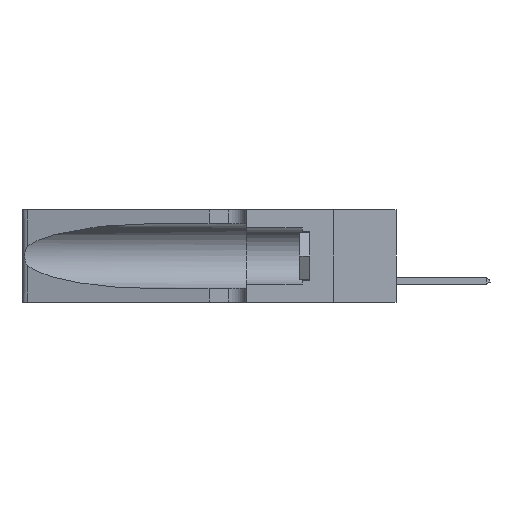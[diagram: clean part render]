
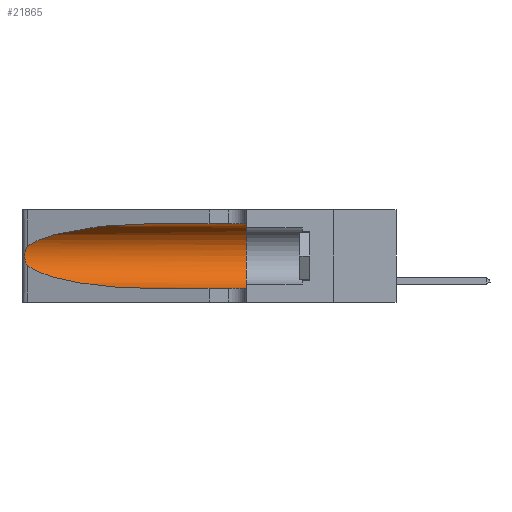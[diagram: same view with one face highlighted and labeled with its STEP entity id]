
A CAD part, left-side view. The second image highlights one B-rep face of the part: STEP entity #21865.
In plain terms, the highlighted cylindrical face has radius 3.308 mm (diameter 6.617 mm), a partial arc.
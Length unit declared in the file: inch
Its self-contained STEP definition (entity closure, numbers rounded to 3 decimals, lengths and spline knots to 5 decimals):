
#190 = AXIS2_PLACEMENT_3D ( 'NONE', #4617, #20242, #4769 ) ;
#362 = CARTESIAN_POINT ( 'NONE',  ( 0.1305, 0.72297, 0.31525 ) ) ;
#919 = CARTESIAN_POINT ( 'NONE',  ( 0.1305, 0.72297, 0.31525 ) ) ;
#1406 = CARTESIAN_POINT ( 'NONE',  ( 0.25487, 1.22718, 0.14631 ) ) ;
#1492 = CARTESIAN_POINT ( 'NONE',  ( 0.26017, 1.23833, 0.17102 ) ) ;
#1553 = CARTESIAN_POINT ( 'NONE',  ( 0.25639, 1.23186, 0.15144 ) ) ;
#1636 = FACE_OUTER_BOUND ( 'NONE', #13879, .T. ) ;
#1815 =( BOUNDED_CURVE ( )  B_SPLINE_CURVE ( 3, ( #362, #12248, #20667, #10382 ),
 .UNSPECIFIED., .F., .T. ) 
 B_SPLINE_CURVE_WITH_KNOTS ( ( 4, 4 ),
 ( 1.5708, 2.84003 ),
 .UNSPECIFIED. ) 
 CURVE ( )  GEOMETRIC_REPRESENTATION_ITEM ( )  RATIONAL_B_SPLINE_CURVE ( ( 1., 0.87, 0.87, 1. ) ) 
 REPRESENTATION_ITEM ( '' )  );
#1851 = VERTEX_POINT ( 'NONE', #919 ) ;
#1918 = ORIENTED_EDGE ( 'NONE', *, *, #15136, .T. ) ;
#2074 = CARTESIAN_POINT ( 'NONE',  ( 0.1305, 1.61858, 0.05475 ) ) ;
#2279 = ORIENTED_EDGE ( 'NONE', *, *, #8762, .F. ) ;
#3175 = B_SPLINE_CURVE_WITH_KNOTS ( 'NONE', 3,
 ( #19698, #7088, #13924, #10709, #17206, #14140, #3721, #17667, #1492, #15080, #20320, #1553, #10096, #13503 ),
 .UNSPECIFIED., .F., .F.,
 ( 4, 2, 2, 2, 2, 2, 4 ),
 ( 0., 0.00027, 0.00053, 0.00107, 0.0016, 0.00187, 0.00214 ),
 .UNSPECIFIED. ) ;
#3478 = VERTEX_POINT ( 'NONE', #22032 ) ;
#3645 = LINE ( 'NONE', #2074, #8427 ) ;
#3721 = CARTESIAN_POINT ( 'NONE',  ( 0.26075, 1.23896, 0.19203 ) ) ;
#4617 = CARTESIAN_POINT ( 'NONE',  ( 0.1305, 0.35, 0.185 ) ) ;
#4769 = DIRECTION ( 'NONE',  ( 0., 0., 1. ) ) ;
#4831 = ORIENTED_EDGE ( 'NONE', *, *, #8500, .T. ) ;
#4931 = DIRECTION ( 'NONE',  ( 0., -1., 0. ) ) ;
#5470 = ORIENTED_EDGE ( 'NONE', *, *, #7664, .T. ) ;
#5628 = CYLINDRICAL_SURFACE ( 'NONE', #19272, 0.13025 ) ;
#5633 = CARTESIAN_POINT ( 'NONE',  ( 0.1305, 1.61858, 0.31525 ) ) ;
#6149 = VERTEX_POINT ( 'NONE', #20934 ) ;
#7088 = CARTESIAN_POINT ( 'NONE',  ( 0.25555, 1.22994, 0.2215 ) ) ;
#7664 = EDGE_CURVE ( 'NONE', #10566, #19313, #8110, .T. ) ;
#7800 = CARTESIAN_POINT ( 'NONE',  ( 0.1305, 0.72297, 0.05475 ) ) ;
#8110 =( BOUNDED_CURVE ( )  B_SPLINE_CURVE ( 3, ( #15711, #19101, #9105, #17372 ),
 .UNSPECIFIED., .F., .F. ) 
 B_SPLINE_CURVE_WITH_KNOTS ( ( 4, 4 ),
 ( 3.44316, 4.71239 ),
 .UNSPECIFIED. ) 
 CURVE ( )  GEOMETRIC_REPRESENTATION_ITEM ( )  RATIONAL_B_SPLINE_CURVE ( ( 1., 0.87, 0.87, 1. ) ) 
 REPRESENTATION_ITEM ( '' )  );
#8427 = VECTOR ( 'NONE', #20833, 39.37008 ) ;
#8500 = EDGE_CURVE ( 'NONE', #19313, #6149, #3645, .T. ) ;
#8762 = EDGE_CURVE ( 'NONE', #1851, #13069, #17769, .T. ) ;
#9105 = CARTESIAN_POINT ( 'NONE',  ( 0.18966, 0.96281, 0.05475 ) ) ;
#10096 = CARTESIAN_POINT ( 'NONE',  ( 0.25555, 1.22993, 0.14849 ) ) ;
#10382 = CARTESIAN_POINT ( 'NONE',  ( 0.25487, 1.22718, 0.22369 ) ) ;
#10566 = VERTEX_POINT ( 'NONE', #1406 ) ;
#10709 = CARTESIAN_POINT ( 'NONE',  ( 0.25787, 1.23484, 0.2124 ) ) ;
#11534 = DIRECTION ( 'NONE',  ( 0., 0., -1. ) ) ;
#12248 = CARTESIAN_POINT ( 'NONE',  ( 0.18966, 0.96281, 0.31525 ) ) ;
#12944 = EDGE_CURVE ( 'NONE', #3478, #10566, #3175, .T. ) ;
#13069 = VERTEX_POINT ( 'NONE', #14559 ) ;
#13503 = CARTESIAN_POINT ( 'NONE',  ( 0.25487, 1.22718, 0.14631 ) ) ;
#13879 = EDGE_LOOP ( 'NONE', ( #1918, #13912, #5470, #4831, #20409, #2279 ) ) ;
#13912 = ORIENTED_EDGE ( 'NONE', *, *, #12944, .T. ) ;
#13924 = CARTESIAN_POINT ( 'NONE',  ( 0.25639, 1.23184, 0.21858 ) ) ;
#14140 = CARTESIAN_POINT ( 'NONE',  ( 0.26018, 1.23835, 0.19895 ) ) ;
#14441 = EDGE_CURVE ( 'NONE', #13069, #6149, #20053, .T. ) ;
#14559 = CARTESIAN_POINT ( 'NONE',  ( 0.1305, 0.35, 0.31525 ) ) ;
#15080 = CARTESIAN_POINT ( 'NONE',  ( 0.25856, 1.23593, 0.16098 ) ) ;
#15099 = CARTESIAN_POINT ( 'NONE',  ( 0.1305, 1.61858, 0.185 ) ) ;
#15136 = EDGE_CURVE ( 'NONE', #1851, #3478, #1815, .T. ) ;
#15711 = CARTESIAN_POINT ( 'NONE',  ( 0.25487, 1.22718, 0.14631 ) ) ;
#17206 = CARTESIAN_POINT ( 'NONE',  ( 0.25854, 1.2359, 0.20912 ) ) ;
#17372 = CARTESIAN_POINT ( 'NONE',  ( 0.1305, 0.72297, 0.05475 ) ) ;
#17566 = DIRECTION ( 'NONE',  ( 0., -1., 0. ) ) ;
#17667 = CARTESIAN_POINT ( 'NONE',  ( 0.26075, 1.23896, 0.178 ) ) ;
#17769 = LINE ( 'NONE', #5633, #21209 ) ;
#19101 = CARTESIAN_POINT ( 'NONE',  ( 0.2373, 1.15595, 0.08982 ) ) ;
#19272 = AXIS2_PLACEMENT_3D ( 'NONE', #15099, #4931, #11534 ) ;
#19313 = VERTEX_POINT ( 'NONE', #7800 ) ;
#19698 = CARTESIAN_POINT ( 'NONE',  ( 0.25487, 1.22718, 0.22369 ) ) ;
#20053 = CIRCLE ( 'NONE', #190, 0.13025 ) ;
#20242 = DIRECTION ( 'NONE',  ( 0., 1., 0. ) ) ;
#20320 = CARTESIAN_POINT ( 'NONE',  ( 0.25789, 1.23486, 0.15765 ) ) ;
#20409 = ORIENTED_EDGE ( 'NONE', *, *, #14441, .F. ) ;
#20667 = CARTESIAN_POINT ( 'NONE',  ( 0.2373, 1.15595, 0.28018 ) ) ;
#20833 = DIRECTION ( 'NONE',  ( 0., -1., 0. ) ) ;
#20934 = CARTESIAN_POINT ( 'NONE',  ( 0.1305, 0.35, 0.05475 ) ) ;
#21209 = VECTOR ( 'NONE', #17566, 39.37008 ) ;
#21865 = ADVANCED_FACE ( 'NONE', ( #1636 ), #5628, .F. ) ;
#22032 = CARTESIAN_POINT ( 'NONE',  ( 0.25487, 1.22718, 0.22369 ) ) ;
